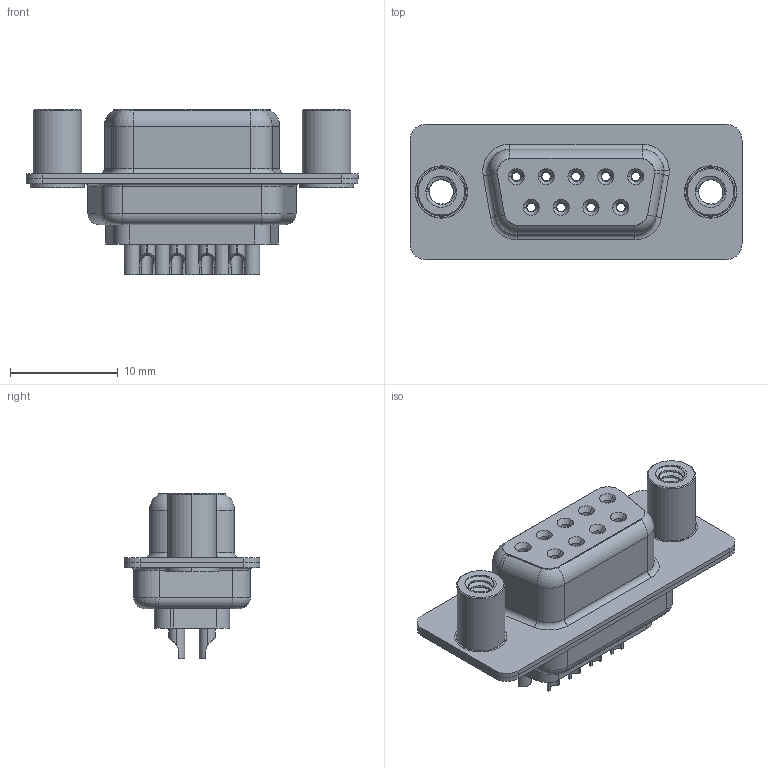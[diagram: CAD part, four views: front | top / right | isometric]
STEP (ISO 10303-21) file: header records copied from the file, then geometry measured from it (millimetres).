
FILE_DESCRIPTION (( 'STEP AP203' ), '1' );
FILE_NAME ('628-009-622-048.STEP', '2020-07-13T22:05:12', ( '' ), ( '' ), 'SwSTEP 2.0', 'SolidWorks 2020', '' );
FILE_SCHEMA (( 'CONFIG_CONTROL_DESIGN' ));
Length unit declared in the file: millimetre
Products named in the file (7): 628-009-622-048; 628 4-40 Threaded Standoff; 628 Shell Rear_09 Contacts; 628 Shell Front_09 Contacts; 628 Contact Row 1_22L; 628 Contact Row 2_22L; 628 Housing_09 LP
Assembly tree (14 placements, depth 2):
  628-009-622-048
    628 Housing_09 LP
    628 Shell Front_09 Contacts
    628 Shell Rear_09 Contacts
    628 Contact Row 1_22L  x5
    628 Contact Row 2_22L  x4
    628 4-40 Threaded Standoff  x2
Bounding box: 30.8 x 12.6 x 15.35 mm (x, y, z)
Volume: 1825.5 mm3; surface area: 4724.3 mm2
Topology: 14 solids, 14 shells, 1114 faces, 2813 edges, 1767 vertices
Faces by surface type: cylinder 390, plane 258, torus 225, bspline 186, cone 55
Entity records: 19867 total; most frequent: CARTESIAN_POINT 6547, DIRECTION 2635, ORIENTED_EDGE 2598, EDGE_CURVE 1299, AXIS2_PLACEMENT_3D 1087, VERTEX_POINT 816, EDGE_LOOP 601, CIRCLE 581
